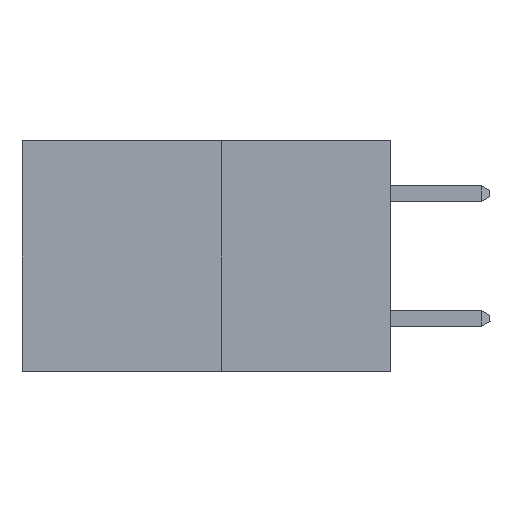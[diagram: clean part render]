
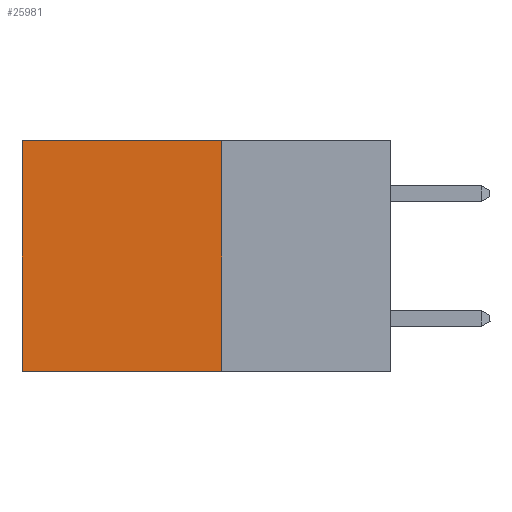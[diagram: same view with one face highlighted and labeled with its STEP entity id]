
A CAD part, left-side view. The second image highlights one B-rep face of the part: STEP entity #25981.
In plain terms, the highlighted planar face has unit normal (-1, 0, 0).
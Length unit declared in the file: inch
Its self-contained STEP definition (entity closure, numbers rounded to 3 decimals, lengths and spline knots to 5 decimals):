
#2103 = VERTEX_POINT ( 'NONE', #18258 ) ;
#3354 = DIRECTION ( 'NONE',  ( 0., 0., -1. ) ) ;
#3694 = LINE ( 'NONE', #15827, #27495 ) ;
#4010 = EDGE_CURVE ( 'NONE', #10016, #26402, #3694, .T. ) ;
#4498 = CARTESIAN_POINT ( 'NONE',  ( 0.277, 0.27, -0.37 ) ) ;
#5916 = ORIENTED_EDGE ( 'NONE', *, *, #10479, .F. ) ;
#6231 = VECTOR ( 'NONE', #18955, 39.37008 ) ;
#6379 = VECTOR ( 'NONE', #26428, 39.37008 ) ;
#6754 = DIRECTION ( 'NONE',  ( 1., 0., 0. ) ) ;
#7541 = ORIENTED_EDGE ( 'NONE', *, *, #18777, .T. ) ;
#7764 = CARTESIAN_POINT ( 'NONE',  ( 0.277, 0.27, -0.37 ) ) ;
#8377 = AXIS2_PLACEMENT_3D ( 'NONE', #4498, #6754, #22427 ) ;
#9120 = ORIENTED_EDGE ( 'NONE', *, *, #23871, .F. ) ;
#9995 = EDGE_LOOP ( 'NONE', ( #7541, #9120, #5916, #19667 ) ) ;
#10016 = VERTEX_POINT ( 'NONE', #11583 ) ;
#10479 = EDGE_CURVE ( 'NONE', #10016, #27079, #11420, .T. ) ;
#10727 = VECTOR ( 'NONE', #3354, 39.37008 ) ;
#11420 = LINE ( 'NONE', #7764, #10727 ) ;
#11583 = CARTESIAN_POINT ( 'NONE',  ( 0.277, 0.27, 0. ) ) ;
#15216 = DIRECTION ( 'NONE',  ( 0., 1., 0. ) ) ;
#15827 = CARTESIAN_POINT ( 'NONE',  ( 0.277, 0.27, 0. ) ) ;
#17271 = CARTESIAN_POINT ( 'NONE',  ( 0.277, 0.59, 0. ) ) ;
#18258 = CARTESIAN_POINT ( 'NONE',  ( 0.277, 0.59, -0.37 ) ) ;
#18777 = EDGE_CURVE ( 'NONE', #26402, #2103, #25498, .T. ) ;
#18955 = DIRECTION ( 'NONE',  ( 0., 0., -1. ) ) ;
#19667 = ORIENTED_EDGE ( 'NONE', *, *, #4010, .T. ) ;
#20185 = PLANE ( 'NONE',  #8377 ) ;
#21706 = FACE_OUTER_BOUND ( 'NONE', #9995, .T. ) ;
#22427 = DIRECTION ( 'NONE',  ( 0., 0., -1. ) ) ;
#23871 = EDGE_CURVE ( 'NONE', #27079, #2103, #24253, .T. ) ;
#24188 = CARTESIAN_POINT ( 'NONE',  ( 0.277, 0.27, -0.37 ) ) ;
#24253 = LINE ( 'NONE', #24188, #6379 ) ;
#25498 = LINE ( 'NONE', #27829, #6231 ) ;
#25981 = ADVANCED_FACE ( 'NONE', ( #21706 ), #20185, .F. ) ;
#26223 = CARTESIAN_POINT ( 'NONE',  ( 0.277, 0.27, -0.37 ) ) ;
#26402 = VERTEX_POINT ( 'NONE', #17271 ) ;
#26428 = DIRECTION ( 'NONE',  ( 0., 1., 0. ) ) ;
#27079 = VERTEX_POINT ( 'NONE', #26223 ) ;
#27495 = VECTOR ( 'NONE', #15216, 39.37008 ) ;
#27829 = CARTESIAN_POINT ( 'NONE',  ( 0.277, 0.59, -0.37 ) ) ;
